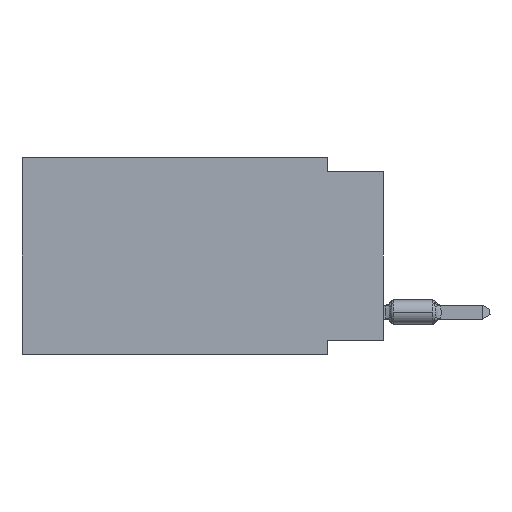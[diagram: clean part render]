
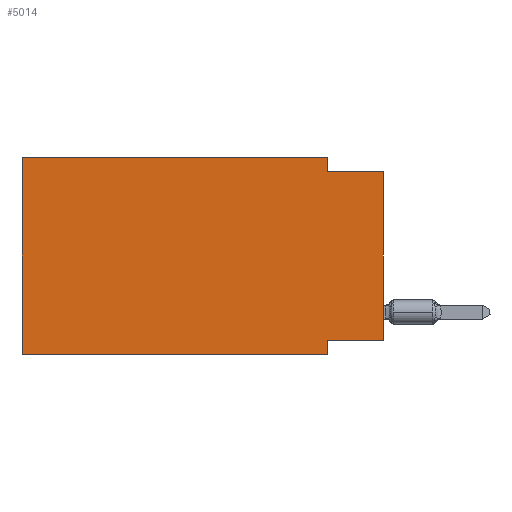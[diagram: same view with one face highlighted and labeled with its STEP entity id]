
A CAD part, left-side view. The second image highlights one B-rep face of the part: STEP entity #5014.
In plain terms, the highlighted planar face has unit normal (-1, 0, 0).
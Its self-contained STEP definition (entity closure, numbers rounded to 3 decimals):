
#305 = VECTOR ( 'NONE', #19534, 1000. ) ;
#921 = CARTESIAN_POINT ( 'NONE',  ( 0., 2.54, -8.89 ) ) ;
#2330 = CARTESIAN_POINT ( 'NONE',  ( 0., 0., 0. ) ) ;
#2603 = ORIENTED_EDGE ( 'NONE', *, *, #23084, .F. ) ;
#3119 = EDGE_CURVE ( 'NONE', #20876, #4107, #6783, .T. ) ;
#3804 = LINE ( 'NONE', #19368, #19378 ) ;
#4107 = VERTEX_POINT ( 'NONE', #13491 ) ;
#4800 = ORIENTED_EDGE ( 'NONE', *, *, #22742, .F. ) ;
#5014 = ADVANCED_FACE ( 'NONE', ( #5402 ), #20693, .F. ) ;
#5402 = FACE_OUTER_BOUND ( 'NONE', #26057, .T. ) ;
#5899 = LINE ( 'NONE', #27923, #14542 ) ;
#6581 = VECTOR ( 'NONE', #22214, 1000. ) ;
#6783 = LINE ( 'NONE', #2330, #15511 ) ;
#7193 = CARTESIAN_POINT ( 'NONE',  ( 0., 2.54, -0.635 ) ) ;
#7573 = DIRECTION ( 'NONE',  ( 1., 0., 0. ) ) ;
#7585 = ORIENTED_EDGE ( 'NONE', *, *, #15880, .F. ) ;
#8139 = VERTEX_POINT ( 'NONE', #18978 ) ;
#8441 = CARTESIAN_POINT ( 'NONE',  ( 0., 16.383, 0. ) ) ;
#9475 = VECTOR ( 'NONE', #24577, 1000. ) ;
#10604 = EDGE_CURVE ( 'NONE', #21577, #11966, #5899, .T. ) ;
#11930 = ORIENTED_EDGE ( 'NONE', *, *, #12100, .F. ) ;
#11966 = VERTEX_POINT ( 'NONE', #7193 ) ;
#12100 = EDGE_CURVE ( 'NONE', #11966, #4107, #3804, .T. ) ;
#12540 = DIRECTION ( 'NONE',  ( 0., 0., -1. ) ) ;
#12602 = DIRECTION ( 'NONE',  ( 0., -1., 0. ) ) ;
#13491 = CARTESIAN_POINT ( 'NONE',  ( 0., 0., -0.635 ) ) ;
#13916 = LINE ( 'NONE', #17803, #9475 ) ;
#14343 = DIRECTION ( 'NONE',  ( 0., 0., -1. ) ) ;
#14542 = VECTOR ( 'NONE', #12540, 1000. ) ;
#14586 = ORIENTED_EDGE ( 'NONE', *, *, #16547, .T. ) ;
#14788 = CARTESIAN_POINT ( 'NONE',  ( 0., 2.54, -8.89 ) ) ;
#15092 = AXIS2_PLACEMENT_3D ( 'NONE', #16090, #7573, #14343 ) ;
#15511 = VECTOR ( 'NONE', #26497, 1000. ) ;
#15880 = EDGE_CURVE ( 'NONE', #20876, #24987, #26943, .T. ) ;
#16090 = CARTESIAN_POINT ( 'NONE',  ( 0., 16.383, 0. ) ) ;
#16306 = ORIENTED_EDGE ( 'NONE', *, *, #3119, .T. ) ;
#16547 = EDGE_CURVE ( 'NONE', #16885, #18079, #21567, .T. ) ;
#16801 = CARTESIAN_POINT ( 'NONE',  ( 0., 2.54, 0. ) ) ;
#16885 = VERTEX_POINT ( 'NONE', #20416 ) ;
#17803 = CARTESIAN_POINT ( 'NONE',  ( 0., 16.383, 0. ) ) ;
#18079 = VERTEX_POINT ( 'NONE', #921 ) ;
#18332 = ORIENTED_EDGE ( 'NONE', *, *, #24611, .F. ) ;
#18639 = ORIENTED_EDGE ( 'NONE', *, *, #10604, .F. ) ;
#18978 = CARTESIAN_POINT ( 'NONE',  ( 0., 16.383, 0. ) ) ;
#19368 = CARTESIAN_POINT ( 'NONE',  ( 0., 0., -0.635 ) ) ;
#19378 = VECTOR ( 'NONE', #12602, 1000. ) ;
#19534 = DIRECTION ( 'NONE',  ( 0., -1., 0. ) ) ;
#20416 = CARTESIAN_POINT ( 'NONE',  ( 0., 16.383, -8.89 ) ) ;
#20693 = PLANE ( 'NONE',  #15092 ) ;
#20876 = VERTEX_POINT ( 'NONE', #25758 ) ;
#21420 = CARTESIAN_POINT ( 'NONE',  ( 0., 16.383, -8.89 ) ) ;
#21567 = LINE ( 'NONE', #21420, #21658 ) ;
#21577 = VERTEX_POINT ( 'NONE', #16801 ) ;
#21658 = VECTOR ( 'NONE', #27885, 1000. ) ;
#22214 = DIRECTION ( 'NONE',  ( 0., 1., 0. ) ) ;
#22742 = EDGE_CURVE ( 'NONE', #24987, #18079, #27074, .T. ) ;
#23084 = EDGE_CURVE ( 'NONE', #16885, #8139, #13916, .T. ) ;
#23567 = LINE ( 'NONE', #8441, #305 ) ;
#24224 = CARTESIAN_POINT ( 'NONE',  ( 0., 0., -8.255 ) ) ;
#24577 = DIRECTION ( 'NONE',  ( 0., 0., 1. ) ) ;
#24611 = EDGE_CURVE ( 'NONE', #8139, #21577, #23567, .T. ) ;
#24782 = DIRECTION ( 'NONE',  ( 0., 0., -1. ) ) ;
#24987 = VERTEX_POINT ( 'NONE', #26454 ) ;
#25532 = VECTOR ( 'NONE', #24782, 1000. ) ;
#25758 = CARTESIAN_POINT ( 'NONE',  ( 0., 0., -8.255 ) ) ;
#26057 = EDGE_LOOP ( 'NONE', ( #16306, #11930, #18639, #18332, #2603, #14586, #4800, #7585 ) ) ;
#26454 = CARTESIAN_POINT ( 'NONE',  ( 0., 2.54, -8.255 ) ) ;
#26497 = DIRECTION ( 'NONE',  ( 0., 0., 1. ) ) ;
#26943 = LINE ( 'NONE', #24224, #6581 ) ;
#27074 = LINE ( 'NONE', #14788, #25532 ) ;
#27885 = DIRECTION ( 'NONE',  ( 0., -1., 0. ) ) ;
#27923 = CARTESIAN_POINT ( 'NONE',  ( 0., 2.54, 0. ) ) ;
